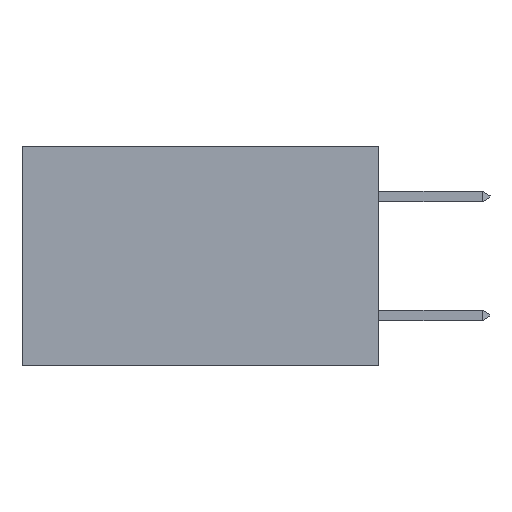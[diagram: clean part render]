
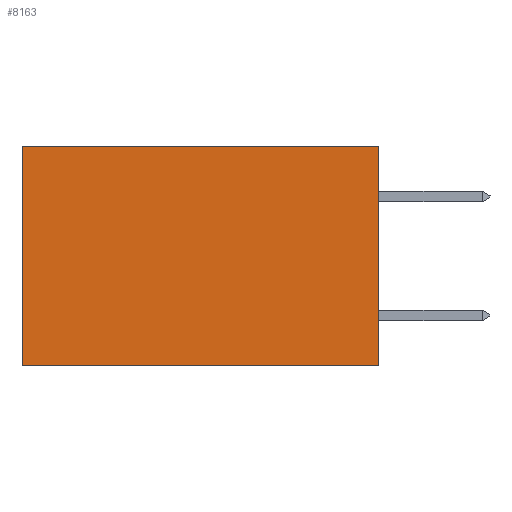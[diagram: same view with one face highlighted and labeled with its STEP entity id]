
A CAD part, left-side view. The second image highlights one B-rep face of the part: STEP entity #8163.
In plain terms, the highlighted planar face has unit normal (-1, 0, 0).
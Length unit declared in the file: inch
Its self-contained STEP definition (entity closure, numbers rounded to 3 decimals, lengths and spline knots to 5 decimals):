
#722 = CARTESIAN_POINT ( 'NONE',  ( 0.2615, 0., 0. ) ) ;
#2748 = DIRECTION ( 'NONE',  ( 0., 1., 0. ) ) ;
#3454 = DIRECTION ( 'NONE',  ( 0., 0., -1. ) ) ;
#4247 = VERTEX_POINT ( 'NONE', #8207 ) ;
#4362 = DIRECTION ( 'NONE',  ( 1., 0., 0. ) ) ;
#4590 = DIRECTION ( 'NONE',  ( 0., 1., 0. ) ) ;
#4752 = EDGE_CURVE ( 'NONE', #9595, #4247, #8583, .T. ) ;
#6136 = AXIS2_PLACEMENT_3D ( 'NONE', #10773, #4362, #15817 ) ;
#6212 = VECTOR ( 'NONE', #3454, 39.37008 ) ;
#6742 = CARTESIAN_POINT ( 'NONE',  ( 0.2615, 0., 0. ) ) ;
#6908 = FACE_OUTER_BOUND ( 'NONE', #13294, .T. ) ;
#6941 = ORIENTED_EDGE ( 'NONE', *, *, #14148, .F. ) ;
#7950 = ORIENTED_EDGE ( 'NONE', *, *, #12343, .T. ) ;
#8042 = LINE ( 'NONE', #722, #11832 ) ;
#8163 = ADVANCED_FACE ( 'NONE', ( #6908 ), #8491, .F. ) ;
#8207 = CARTESIAN_POINT ( 'NONE',  ( 0.2615, 0.6, -0.37 ) ) ;
#8491 = PLANE ( 'NONE',  #6136 ) ;
#8583 = LINE ( 'NONE', #16392, #13879 ) ;
#9152 = LINE ( 'NONE', #9232, #13730 ) ;
#9232 = CARTESIAN_POINT ( 'NONE',  ( 0.2615, 0., -0.37 ) ) ;
#9595 = VERTEX_POINT ( 'NONE', #14033 ) ;
#9688 = VERTEX_POINT ( 'NONE', #6742 ) ;
#9706 = CARTESIAN_POINT ( 'NONE',  ( 0.2615, 0., -0.37 ) ) ;
#10428 = ORIENTED_EDGE ( 'NONE', *, *, #13308, .F. ) ;
#10773 = CARTESIAN_POINT ( 'NONE',  ( 0.2615, 0., -0.37 ) ) ;
#11585 = CARTESIAN_POINT ( 'NONE',  ( 0.2615, 0., -0.37 ) ) ;
#11832 = VECTOR ( 'NONE', #4590, 39.37008 ) ;
#12343 = EDGE_CURVE ( 'NONE', #9688, #9595, #8042, .T. ) ;
#13294 = EDGE_LOOP ( 'NONE', ( #14836, #6941, #10428, #7950 ) ) ;
#13308 = EDGE_CURVE ( 'NONE', #9688, #13876, #13787, .T. ) ;
#13730 = VECTOR ( 'NONE', #2748, 39.37008 ) ;
#13787 = LINE ( 'NONE', #9706, #6212 ) ;
#13876 = VERTEX_POINT ( 'NONE', #11585 ) ;
#13879 = VECTOR ( 'NONE', #14816, 39.37008 ) ;
#14033 = CARTESIAN_POINT ( 'NONE',  ( 0.2615, 0.6, 0. ) ) ;
#14148 = EDGE_CURVE ( 'NONE', #13876, #4247, #9152, .T. ) ;
#14816 = DIRECTION ( 'NONE',  ( 0., 0., -1. ) ) ;
#14836 = ORIENTED_EDGE ( 'NONE', *, *, #4752, .T. ) ;
#15817 = DIRECTION ( 'NONE',  ( 0., 0., -1. ) ) ;
#16392 = CARTESIAN_POINT ( 'NONE',  ( 0.2615, 0.6, -0.37 ) ) ;
